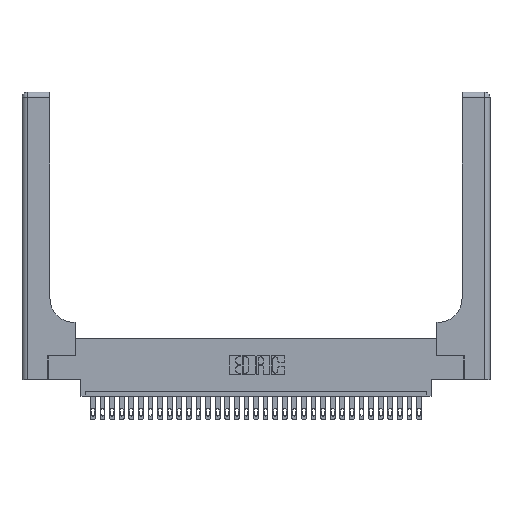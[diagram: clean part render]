
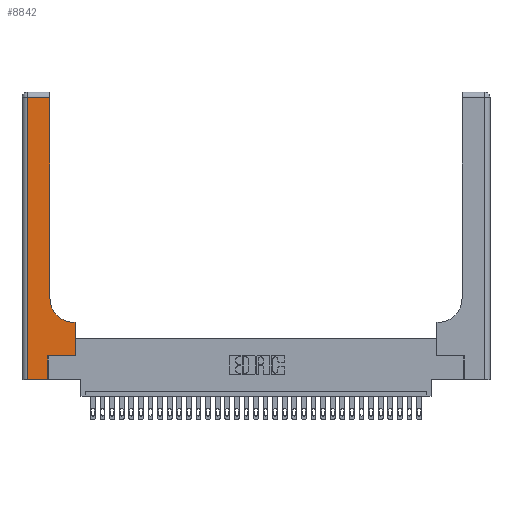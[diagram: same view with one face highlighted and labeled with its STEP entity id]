
A CAD part, top view. The second image highlights one B-rep face of the part: STEP entity #8842.
In plain terms, the highlighted planar face has unit normal (0, 0, 1).
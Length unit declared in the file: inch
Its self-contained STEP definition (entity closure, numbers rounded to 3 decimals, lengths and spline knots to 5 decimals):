
#448 = DIRECTION ( 'NONE',  ( 0., 1., 0. ) ) ;
#662 = CARTESIAN_POINT ( 'NONE',  ( 0.269, 0., 0.37 ) ) ;
#827 = CARTESIAN_POINT ( 'NONE',  ( 0.06, 2.94, 0.37 ) ) ;
#1322 = DIRECTION ( 'NONE',  ( -1., 0., 0. ) ) ;
#1567 = VERTEX_POINT ( 'NONE', #827 ) ;
#1665 = CARTESIAN_POINT ( 'NONE',  ( 0.5585, 0.25, 0.37 ) ) ;
#2310 = VECTOR ( 'NONE', #6350, 39.37008 ) ;
#3025 = VERTEX_POINT ( 'NONE', #27903 ) ;
#3081 = LINE ( 'NONE', #16119, #2310 ) ;
#3574 = CARTESIAN_POINT ( 'NONE',  ( 0.269, 0.25, 0.37 ) ) ;
#5130 = VECTOR ( 'NONE', #18020, 39.37008 ) ;
#5162 = CARTESIAN_POINT ( 'NONE',  ( 0.2915, 0.85, 0.37 ) ) ;
#6350 = DIRECTION ( 'NONE',  ( 0., 1., 0. ) ) ;
#7353 = ORIENTED_EDGE ( 'NONE', *, *, #10983, .T. ) ;
#8825 = LINE ( 'NONE', #31415, #19776 ) ;
#8842 = ADVANCED_FACE ( 'NONE', ( #27148 ), #15757, .F. ) ;
#8896 = EDGE_CURVE ( 'NONE', #24995, #18796, #11870, .T. ) ;
#8908 = DIRECTION ( 'NONE',  ( 1., 0., 0. ) ) ;
#8936 = CARTESIAN_POINT ( 'NONE',  ( 0.06, 3., 0.37 ) ) ;
#9889 = ORIENTED_EDGE ( 'NONE', *, *, #25585, .T. ) ;
#9952 = AXIS2_PLACEMENT_3D ( 'NONE', #27799, #12769, #31014 ) ;
#10477 = ORIENTED_EDGE ( 'NONE', *, *, #19417, .T. ) ;
#10983 = EDGE_CURVE ( 'NONE', #15801, #24995, #11266, .T. ) ;
#11004 = DIRECTION ( 'NONE',  ( 0., -1., 0. ) ) ;
#11266 = LINE ( 'NONE', #29111, #14035 ) ;
#11351 = CARTESIAN_POINT ( 'NONE',  ( 0.5585, 0.25, 0.37 ) ) ;
#11397 = ORIENTED_EDGE ( 'NONE', *, *, #26709, .T. ) ;
#11870 = LINE ( 'NONE', #11351, #24408 ) ;
#12330 = EDGE_CURVE ( 'NONE', #15408, #15067, #27697, .T. ) ;
#12769 = DIRECTION ( 'NONE',  ( 0., 0., -1. ) ) ;
#13510 = CARTESIAN_POINT ( 'NONE',  ( 0., 2.94, 0.37 ) ) ;
#13533 = CARTESIAN_POINT ( 'NONE',  ( 0., 3., 0.37 ) ) ;
#13755 = ORIENTED_EDGE ( 'NONE', *, *, #23521, .T. ) ;
#14035 = VECTOR ( 'NONE', #29004, 39.37008 ) ;
#14417 = ORIENTED_EDGE ( 'NONE', *, *, #19265, .T. ) ;
#14585 = CARTESIAN_POINT ( 'NONE',  ( 0.5415, 0.6, 0.37 ) ) ;
#15067 = VERTEX_POINT ( 'NONE', #5162 ) ;
#15408 = VERTEX_POINT ( 'NONE', #14585 ) ;
#15757 = PLANE ( 'NONE',  #22204 ) ;
#15801 = VERTEX_POINT ( 'NONE', #3574 ) ;
#16119 = CARTESIAN_POINT ( 'NONE',  ( 0.2915, 3., 0.37 ) ) ;
#18020 = DIRECTION ( 'NONE',  ( -1., 0., 0. ) ) ;
#18152 = DIRECTION ( 'NONE',  ( 0., 0., -1. ) ) ;
#18259 = DIRECTION ( 'NONE',  ( -1., 0., 0. ) ) ;
#18796 = VERTEX_POINT ( 'NONE', #21117 ) ;
#18861 = CARTESIAN_POINT ( 'NONE',  ( 0., 0., 0.37 ) ) ;
#19148 = LINE ( 'NONE', #8936, #21505 ) ;
#19265 = EDGE_CURVE ( 'NONE', #23055, #15801, #26686, .T. ) ;
#19417 = EDGE_CURVE ( 'NONE', #15067, #3025, #3081, .T. ) ;
#19765 = CARTESIAN_POINT ( 'NONE',  ( 0.269, 0., 0.37 ) ) ;
#19776 = VECTOR ( 'NONE', #1322, 39.37008 ) ;
#21117 = CARTESIAN_POINT ( 'NONE',  ( 0.5585, 0.6, 0.37 ) ) ;
#21505 = VECTOR ( 'NONE', #11004, 39.37008 ) ;
#22204 = AXIS2_PLACEMENT_3D ( 'NONE', #13533, #18152, #18259 ) ;
#22375 = LINE ( 'NONE', #18861, #29090 ) ;
#22782 = EDGE_CURVE ( 'NONE', #3025, #1567, #29534, .T. ) ;
#23055 = VERTEX_POINT ( 'NONE', #19765 ) ;
#23521 = EDGE_CURVE ( 'NONE', #18796, #15408, #8825, .T. ) ;
#24132 = ORIENTED_EDGE ( 'NONE', *, *, #22782, .T. ) ;
#24408 = VECTOR ( 'NONE', #31683, 39.37008 ) ;
#24995 = VERTEX_POINT ( 'NONE', #1665 ) ;
#25585 = EDGE_CURVE ( 'NONE', #28817, #23055, #22375, .T. ) ;
#25653 = EDGE_LOOP ( 'NONE', ( #10477, #24132, #11397, #9889, #14417, #7353, #25992, #13755, #27733 ) ) ;
#25992 = ORIENTED_EDGE ( 'NONE', *, *, #8896, .T. ) ;
#26686 = LINE ( 'NONE', #662, #30237 ) ;
#26709 = EDGE_CURVE ( 'NONE', #1567, #28817, #19148, .T. ) ;
#27148 = FACE_OUTER_BOUND ( 'NONE', #25653, .T. ) ;
#27697 = CIRCLE ( 'NONE', #9952, 0.25 ) ;
#27733 = ORIENTED_EDGE ( 'NONE', *, *, #12330, .T. ) ;
#27799 = CARTESIAN_POINT ( 'NONE',  ( 0.5415, 0.85, 0.37 ) ) ;
#27903 = CARTESIAN_POINT ( 'NONE',  ( 0.2915, 2.94, 0.37 ) ) ;
#28817 = VERTEX_POINT ( 'NONE', #30247 ) ;
#29004 = DIRECTION ( 'NONE',  ( 1., 0., 0. ) ) ;
#29090 = VECTOR ( 'NONE', #8908, 39.37008 ) ;
#29111 = CARTESIAN_POINT ( 'NONE',  ( 0.269, 0.25, 0.37 ) ) ;
#29534 = LINE ( 'NONE', #13510, #5130 ) ;
#30237 = VECTOR ( 'NONE', #448, 39.37008 ) ;
#30247 = CARTESIAN_POINT ( 'NONE',  ( 0.06, 0., 0.37 ) ) ;
#31014 = DIRECTION ( 'NONE',  ( 1., 0., 0. ) ) ;
#31415 = CARTESIAN_POINT ( 'NONE',  ( 0.2915, 0.6, 0.37 ) ) ;
#31683 = DIRECTION ( 'NONE',  ( 0., 1., 0. ) ) ;
